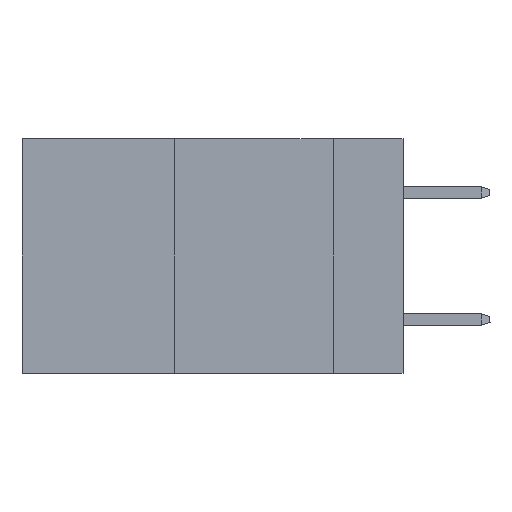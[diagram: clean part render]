
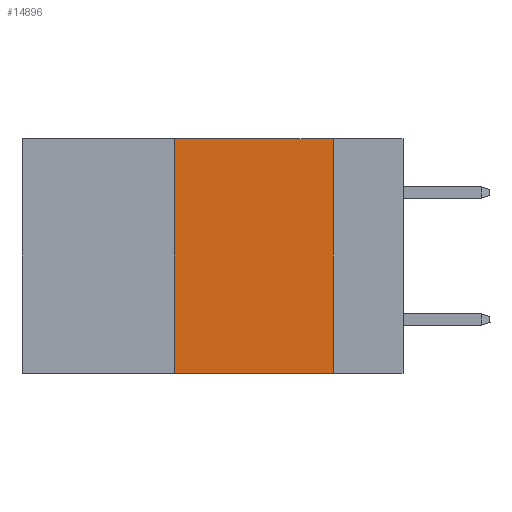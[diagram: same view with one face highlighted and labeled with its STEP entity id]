
A CAD part, left-side view. The second image highlights one B-rep face of the part: STEP entity #14896.
In plain terms, the highlighted planar face has unit normal (-1, 0, 0).
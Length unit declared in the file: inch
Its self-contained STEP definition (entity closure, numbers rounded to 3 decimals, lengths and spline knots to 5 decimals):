
#1143 = CARTESIAN_POINT ( 'NONE',  ( 0., 0.6, 0. ) ) ;
#2069 = LINE ( 'NONE', #5995, #15450 ) ;
#4255 = AXIS2_PLACEMENT_3D ( 'NONE', #1143, #24088, #5614 ) ;
#4580 = LINE ( 'NONE', #21013, #8550 ) ;
#5614 = DIRECTION ( 'NONE',  ( 0., 0., -1. ) ) ;
#5995 = CARTESIAN_POINT ( 'NONE',  ( 0., 0.6, 0. ) ) ;
#6762 = ORIENTED_EDGE ( 'NONE', *, *, #16608, .T. ) ;
#8249 = DIRECTION ( 'NONE',  ( 0., 0., -1. ) ) ;
#8550 = VECTOR ( 'NONE', #18979, 39.37008 ) ;
#9386 = ORIENTED_EDGE ( 'NONE', *, *, #19987, .F. ) ;
#9482 = ORIENTED_EDGE ( 'NONE', *, *, #9539, .F. ) ;
#9539 = EDGE_CURVE ( 'NONE', #14998, #12970, #4580, .T. ) ;
#9619 = LINE ( 'NONE', #13673, #18008 ) ;
#9862 = EDGE_CURVE ( 'NONE', #12970, #11260, #2069, .T. ) ;
#11260 = VERTEX_POINT ( 'NONE', #21825 ) ;
#12328 = VERTEX_POINT ( 'NONE', #24741 ) ;
#12437 = LINE ( 'NONE', #22153, #16794 ) ;
#12970 = VERTEX_POINT ( 'NONE', #19896 ) ;
#13409 = DIRECTION ( 'NONE',  ( 0., -1., 0. ) ) ;
#13673 = CARTESIAN_POINT ( 'NONE',  ( 0., 0.6, -0.37 ) ) ;
#14896 = ADVANCED_FACE ( 'NONE', ( #23961 ), #21787, .F. ) ;
#14998 = VERTEX_POINT ( 'NONE', #16221 ) ;
#15450 = VECTOR ( 'NONE', #22450, 39.37008 ) ;
#16221 = CARTESIAN_POINT ( 'NONE',  ( 0., 0.36, -0.37 ) ) ;
#16608 = EDGE_CURVE ( 'NONE', #14998, #12328, #9619, .T. ) ;
#16794 = VECTOR ( 'NONE', #8249, 39.37008 ) ;
#17400 = EDGE_LOOP ( 'NONE', ( #9386, #21911, #9482, #6762 ) ) ;
#18008 = VECTOR ( 'NONE', #13409, 39.37008 ) ;
#18979 = DIRECTION ( 'NONE',  ( 0., 0., 1. ) ) ;
#19896 = CARTESIAN_POINT ( 'NONE',  ( 0., 0.36, 0. ) ) ;
#19987 = EDGE_CURVE ( 'NONE', #11260, #12328, #12437, .T. ) ;
#21013 = CARTESIAN_POINT ( 'NONE',  ( 0., 0.36, 0. ) ) ;
#21787 = PLANE ( 'NONE',  #4255 ) ;
#21825 = CARTESIAN_POINT ( 'NONE',  ( 0., 0.11, 0. ) ) ;
#21911 = ORIENTED_EDGE ( 'NONE', *, *, #9862, .F. ) ;
#22153 = CARTESIAN_POINT ( 'NONE',  ( 0., 0.11, 0. ) ) ;
#22450 = DIRECTION ( 'NONE',  ( 0., -1., 0. ) ) ;
#23961 = FACE_OUTER_BOUND ( 'NONE', #17400, .T. ) ;
#24088 = DIRECTION ( 'NONE',  ( 1., 0., 0. ) ) ;
#24741 = CARTESIAN_POINT ( 'NONE',  ( 0., 0.11, -0.37 ) ) ;
